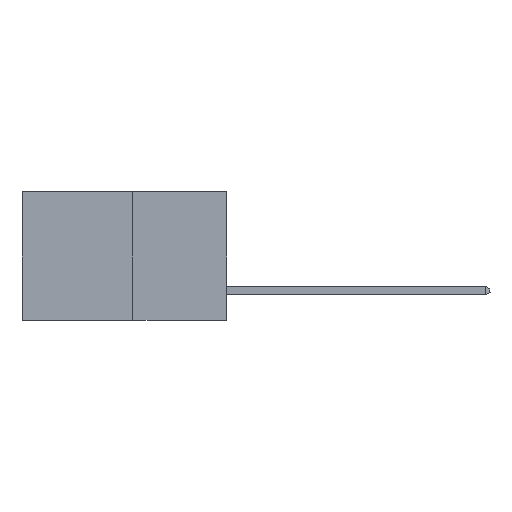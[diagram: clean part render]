
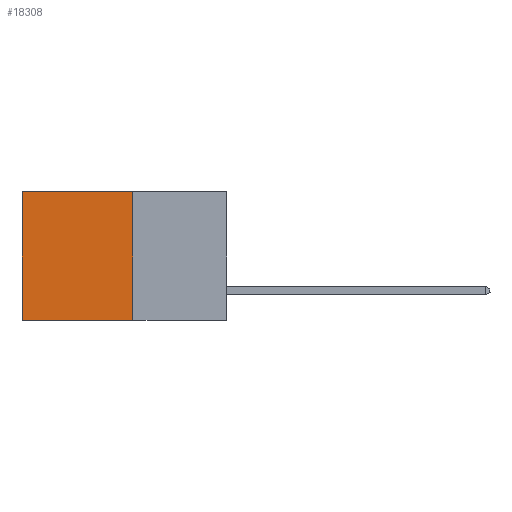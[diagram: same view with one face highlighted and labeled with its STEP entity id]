
A CAD part, left-side view. The second image highlights one B-rep face of the part: STEP entity #18308.
In plain terms, the highlighted planar face has unit normal (-1, 0, 0).
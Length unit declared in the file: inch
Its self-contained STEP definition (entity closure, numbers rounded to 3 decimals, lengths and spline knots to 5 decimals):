
#973 = LINE ( 'NONE', #15080, #18031 ) ;
#2370 = VERTEX_POINT ( 'NONE', #20138 ) ;
#2405 = LINE ( 'NONE', #6387, #14560 ) ;
#2515 = ORIENTED_EDGE ( 'NONE', *, *, #16008, .T. ) ;
#2851 = EDGE_CURVE ( 'NONE', #17292, #4890, #5515, .T. ) ;
#3411 = DIRECTION ( 'NONE',  ( 0., 1., 0. ) ) ;
#3772 = LINE ( 'NONE', #7092, #8078 ) ;
#4890 = VERTEX_POINT ( 'NONE', #11773 ) ;
#5515 = LINE ( 'NONE', #19320, #13413 ) ;
#6184 = ORIENTED_EDGE ( 'NONE', *, *, #14648, .F. ) ;
#6189 = DIRECTION ( 'NONE',  ( 0., 0., -1. ) ) ;
#6387 = CARTESIAN_POINT ( 'NONE',  ( 0.277, 0.27, -0.37 ) ) ;
#7027 = CARTESIAN_POINT ( 'NONE',  ( 0.277, 0.27, 0. ) ) ;
#7092 = CARTESIAN_POINT ( 'NONE',  ( 0.277, 0.27, -0.37 ) ) ;
#7359 = CARTESIAN_POINT ( 'NONE',  ( 0.277, 0.59, -0.37 ) ) ;
#8078 = VECTOR ( 'NONE', #17829, 39.37008 ) ;
#8243 = ORIENTED_EDGE ( 'NONE', *, *, #11767, .F. ) ;
#8744 = AXIS2_PLACEMENT_3D ( 'NONE', #20029, #15539, #6189 ) ;
#10575 = ORIENTED_EDGE ( 'NONE', *, *, #2851, .T. ) ;
#10776 = FACE_OUTER_BOUND ( 'NONE', #12842, .T. ) ;
#11767 = EDGE_CURVE ( 'NONE', #2370, #19363, #2405, .T. ) ;
#11773 = CARTESIAN_POINT ( 'NONE',  ( 0.277, 0.59, 0. ) ) ;
#12842 = EDGE_LOOP ( 'NONE', ( #2515, #8243, #6184, #10575 ) ) ;
#13413 = VECTOR ( 'NONE', #3411, 39.37008 ) ;
#14013 = PLANE ( 'NONE',  #8744 ) ;
#14199 = DIRECTION ( 'NONE',  ( 0., 1., 0. ) ) ;
#14560 = VECTOR ( 'NONE', #14199, 39.37008 ) ;
#14648 = EDGE_CURVE ( 'NONE', #17292, #2370, #3772, .T. ) ;
#15080 = CARTESIAN_POINT ( 'NONE',  ( 0.277, 0.59, -0.37 ) ) ;
#15539 = DIRECTION ( 'NONE',  ( 1., 0., 0. ) ) ;
#16008 = EDGE_CURVE ( 'NONE', #4890, #19363, #973, .T. ) ;
#16550 = DIRECTION ( 'NONE',  ( 0., 0., -1. ) ) ;
#17292 = VERTEX_POINT ( 'NONE', #7027 ) ;
#17829 = DIRECTION ( 'NONE',  ( 0., 0., -1. ) ) ;
#18031 = VECTOR ( 'NONE', #16550, 39.37008 ) ;
#18308 = ADVANCED_FACE ( 'NONE', ( #10776 ), #14013, .F. ) ;
#19320 = CARTESIAN_POINT ( 'NONE',  ( 0.277, 0.27, 0. ) ) ;
#19363 = VERTEX_POINT ( 'NONE', #7359 ) ;
#20029 = CARTESIAN_POINT ( 'NONE',  ( 0.277, 0.27, -0.37 ) ) ;
#20138 = CARTESIAN_POINT ( 'NONE',  ( 0.277, 0.27, -0.37 ) ) ;
